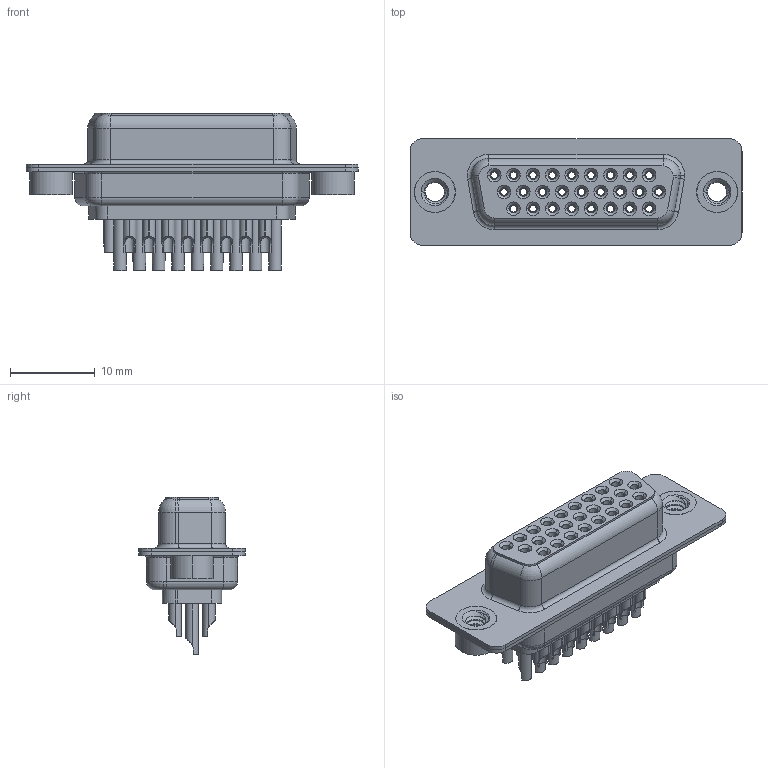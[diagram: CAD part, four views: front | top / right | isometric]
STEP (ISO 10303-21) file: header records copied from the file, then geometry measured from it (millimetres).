
FILE_DESCRIPTION (( 'STEP AP203' ), '1' );
FILE_NAME ('638-026-632-262.STEP', '2020-07-18T21:55:30', ( '' ), ( '' ), 'SwSTEP 2.0', 'SolidWorks 2020', '' );
FILE_SCHEMA (( 'CONFIG_CONTROL_DESIGN' ));
Length unit declared in the file: millimetre
Products named in the file (8): 638 Shell Rear_26 Contacts; 638 4-40 Threaded Rivet; 638 Shell Front_26 Contacts; 638 Housing_26 Contacts; 638 Contact Row 3_32; 638-026-632-262; 638 Contact Row 1_32; 638 Contact Row 2_32
Assembly tree (31 placements, depth 2):
  638-026-632-262
    638 Housing_26 Contacts
    638 Shell Front_26 Contacts
    638 Shell Rear_26 Contacts
    638 Contact Row 1_32  x9
    638 Contact Row 2_32  x9
    638 Contact Row 3_32  x8
    638 4-40 Threaded Rivet  x2
Bounding box: 39.19 x 12.6 x 18.6 mm (x, y, z)
Volume: 2261.8 mm3; surface area: 8768.3 mm2
Topology: 31 solids, 31 shells, 2593 faces, 6561 edges, 4119 vertices
Faces by surface type: cylinder 787, plane 613, bspline 526, torus 525, cone 142
Entity records: 28936 total; most frequent: CARTESIAN_POINT 8517, DIRECTION 4129, ORIENTED_EDGE 3852, EDGE_CURVE 1926, AXIS2_PLACEMENT_3D 1728, VERTEX_POINT 1215, EDGE_LOOP 965, CIRCLE 945
